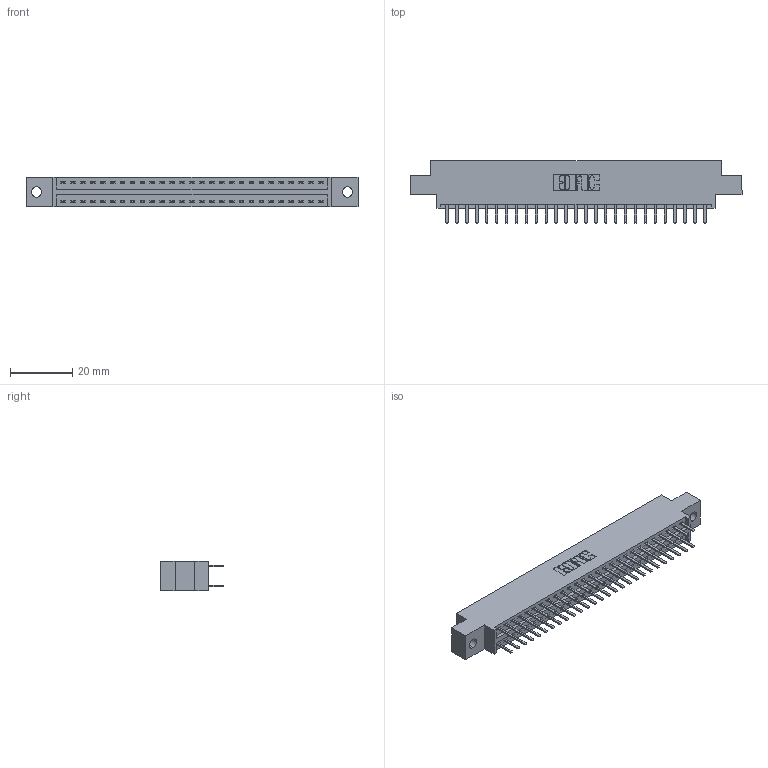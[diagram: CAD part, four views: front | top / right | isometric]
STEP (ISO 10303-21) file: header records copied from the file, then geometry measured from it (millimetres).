
FILE_DESCRIPTION (( 'STEP AP203' ), '1' );
FILE_NAME ('346-054-520-802.STEP', '2022-05-21T02:43:41', ( '' ), ( '' ), 'SwSTEP 2.0', 'SolidWorks 2020', '' );
FILE_SCHEMA (( 'CONFIG_CONTROL_DESIGN' ));
Length unit declared in the file: inch
Products named in the file (3): 346 Part_0.170 Offset - 0.128 Dia; 345-292-001_345-293-120; 346-054-520-802
Assembly tree (55 placements, depth 2):
  346-054-520-802
    346 Part_0.170 Offset - 0.128 Dia
    345-292-001_345-293-120  x54
Bounding box: 106.3 x 20.02 x 9.4 mm (x, y, z)
Volume: 10033.9 mm3; surface area: 13411.3 mm2
Topology: 55 solids, 55 shells, 3150 faces, 9143 edges, 5950 vertices
Faces by surface type: plane 2078, cylinder 1072
Entity records: 19889 total; most frequent: CARTESIAN_POINT 3312, ORIENTED_EDGE 3234, DIRECTION 2957, EDGE_CURVE 1617, LINE 1373, VECTOR 1373, VERTEX_POINT 1074, AXIS2_PLACEMENT_3D 792
